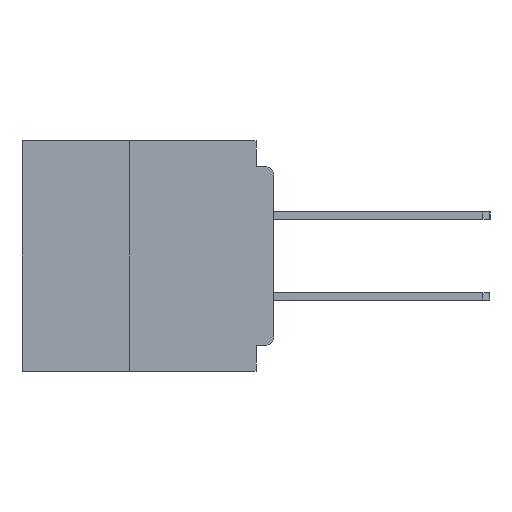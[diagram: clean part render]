
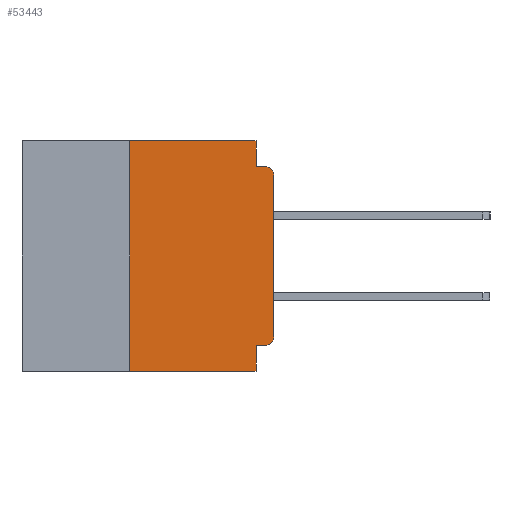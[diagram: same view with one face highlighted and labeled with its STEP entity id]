
A CAD part, left-side view. The second image highlights one B-rep face of the part: STEP entity #53443.
In plain terms, the highlighted planar face has unit normal (-1, 0, 0).
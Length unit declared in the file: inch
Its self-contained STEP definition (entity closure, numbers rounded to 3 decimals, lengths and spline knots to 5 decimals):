
#394 = VECTOR ( 'NONE', #37927, 39.37008 ) ;
#3602 = EDGE_CURVE ( 'NONE', #53124, #41101, #30416, .T. ) ;
#3615 = VECTOR ( 'NONE', #16809, 39.37008 ) ;
#4564 = PLANE ( 'NONE',  #59896 ) ;
#5155 = DIRECTION ( 'NONE',  ( 0., 0., 1. ) ) ;
#5938 = AXIS2_PLACEMENT_3D ( 'NONE', #44408, #13961, #49555 ) ;
#7149 = ORIENTED_EDGE ( 'NONE', *, *, #55955, .F. ) ;
#7468 = ORIENTED_EDGE ( 'NONE', *, *, #63781, .F. ) ;
#8582 = LINE ( 'NONE', #30007, #11817 ) ;
#8598 = VECTOR ( 'NONE', #38823, 39.37008 ) ;
#8826 = EDGE_CURVE ( 'NONE', #54804, #32072, #51766, .T. ) ;
#9048 = EDGE_CURVE ( 'NONE', #41101, #62053, #10284, .T. ) ;
#9780 = CARTESIAN_POINT ( 'NONE',  ( 0., 0.031, -0.355 ) ) ;
#10227 = LINE ( 'NONE', #23734, #8598 ) ;
#10284 = CIRCLE ( 'NONE', #5938, 0.015 ) ;
#11650 = CARTESIAN_POINT ( 'NONE',  ( 0., 0., -0.045 ) ) ;
#11817 = VECTOR ( 'NONE', #65470, 39.37008 ) ;
#11975 = ORIENTED_EDGE ( 'NONE', *, *, #19050, .F. ) ;
#13444 = CARTESIAN_POINT ( 'NONE',  ( 0., 0.031, -0.4 ) ) ;
#13961 = DIRECTION ( 'NONE',  ( -1., 0., 0. ) ) ;
#16021 = ORIENTED_EDGE ( 'NONE', *, *, #52593, .F. ) ;
#16647 = CARTESIAN_POINT ( 'NONE',  ( 0., 0.25, 0. ) ) ;
#16809 = DIRECTION ( 'NONE',  ( 0., -1., 0. ) ) ;
#16844 = VECTOR ( 'NONE', #5155, 39.37008 ) ;
#17705 = CARTESIAN_POINT ( 'NONE',  ( 0., 0.015, -0.34 ) ) ;
#19050 = EDGE_CURVE ( 'NONE', #55269, #35301, #8582, .T. ) ;
#22623 = ORIENTED_EDGE ( 'NONE', *, *, #8826, .T. ) ;
#22853 = DIRECTION ( 'NONE',  ( 0., 0., -1. ) ) ;
#23224 = ORIENTED_EDGE ( 'NONE', *, *, #56263, .F. ) ;
#23734 = CARTESIAN_POINT ( 'NONE',  ( 0., 0.031, 0. ) ) ;
#25204 = DIRECTION ( 'NONE',  ( 1., 0., 0. ) ) ;
#26945 = DIRECTION ( 'NONE',  ( 0., -1., 0. ) ) ;
#28700 = ORIENTED_EDGE ( 'NONE', *, *, #57626, .T. ) ;
#28778 = CARTESIAN_POINT ( 'NONE',  ( 0., 0.031, 0. ) ) ;
#29276 = ORIENTED_EDGE ( 'NONE', *, *, #52467, .F. ) ;
#30007 = CARTESIAN_POINT ( 'NONE',  ( 0., 0., -0.355 ) ) ;
#30416 = LINE ( 'NONE', #55993, #16844 ) ;
#30846 = LINE ( 'NONE', #11650, #3615 ) ;
#31445 = CARTESIAN_POINT ( 'NONE',  ( 0., 0.015, -0.045 ) ) ;
#31579 = CARTESIAN_POINT ( 'NONE',  ( 0., 0., -0.06 ) ) ;
#32072 = VERTEX_POINT ( 'NONE', #13444 ) ;
#32829 = CARTESIAN_POINT ( 'NONE',  ( 0., 0.25, -0.4 ) ) ;
#34481 = VERTEX_POINT ( 'NONE', #64232 ) ;
#35301 = VERTEX_POINT ( 'NONE', #9780 ) ;
#37617 = LINE ( 'NONE', #61578, #49532 ) ;
#37927 = DIRECTION ( 'NONE',  ( 0., 0., 1. ) ) ;
#37977 = LINE ( 'NONE', #32829, #394 ) ;
#38823 = DIRECTION ( 'NONE',  ( 0., 0., -1. ) ) ;
#41101 = VERTEX_POINT ( 'NONE', #31579 ) ;
#41611 = VECTOR ( 'NONE', #58799, 39.37008 ) ;
#42228 = CARTESIAN_POINT ( 'NONE',  ( 0., 0.437, -0.4 ) ) ;
#44310 = AXIS2_PLACEMENT_3D ( 'NONE', #17705, #53309, #22853 ) ;
#44408 = CARTESIAN_POINT ( 'NONE',  ( 0., 0.015, -0.06 ) ) ;
#44816 = VERTEX_POINT ( 'NONE', #16647 ) ;
#46308 = DIRECTION ( 'NONE',  ( 0., -1., 0. ) ) ;
#48862 = VERTEX_POINT ( 'NONE', #28778 ) ;
#49532 = VECTOR ( 'NONE', #46308, 39.37008 ) ;
#49555 = DIRECTION ( 'NONE',  ( 0., 0., -1. ) ) ;
#51372 = FACE_OUTER_BOUND ( 'NONE', #62338, .T. ) ;
#51766 = LINE ( 'NONE', #42228, #65213 ) ;
#52467 = EDGE_CURVE ( 'NONE', #34481, #62053, #30846, .T. ) ;
#52593 = EDGE_CURVE ( 'NONE', #54804, #44816, #37977, .T. ) ;
#53124 = VERTEX_POINT ( 'NONE', #53235 ) ;
#53235 = CARTESIAN_POINT ( 'NONE',  ( 0., 0., -0.34 ) ) ;
#53309 = DIRECTION ( 'NONE',  ( -1., 0., 0. ) ) ;
#53377 = CARTESIAN_POINT ( 'NONE',  ( 0., 0.015, -0.355 ) ) ;
#53443 = ADVANCED_FACE ( 'NONE', ( #51372 ), #4564, .F. ) ;
#53732 = CARTESIAN_POINT ( 'NONE',  ( 0., 0.031, -0.4 ) ) ;
#54699 = ORIENTED_EDGE ( 'NONE', *, *, #9048, .T. ) ;
#54804 = VERTEX_POINT ( 'NONE', #56774 ) ;
#55163 = LINE ( 'NONE', #53732, #41611 ) ;
#55269 = VERTEX_POINT ( 'NONE', #53377 ) ;
#55626 = CARTESIAN_POINT ( 'NONE',  ( 0., 0.437, 0. ) ) ;
#55955 = EDGE_CURVE ( 'NONE', #35301, #32072, #55163, .T. ) ;
#55993 = CARTESIAN_POINT ( 'NONE',  ( 0., 0., 0. ) ) ;
#56263 = EDGE_CURVE ( 'NONE', #44816, #48862, #37617, .T. ) ;
#56774 = CARTESIAN_POINT ( 'NONE',  ( 0., 0.25, -0.4 ) ) ;
#57626 = EDGE_CURVE ( 'NONE', #55269, #53124, #62788, .T. ) ;
#58799 = DIRECTION ( 'NONE',  ( 0., 0., -1. ) ) ;
#59896 = AXIS2_PLACEMENT_3D ( 'NONE', #55626, #25204, #60673 ) ;
#60195 = ORIENTED_EDGE ( 'NONE', *, *, #3602, .T. ) ;
#60673 = DIRECTION ( 'NONE',  ( 0., 0., -1. ) ) ;
#61578 = CARTESIAN_POINT ( 'NONE',  ( 0., 0.437, 0. ) ) ;
#62053 = VERTEX_POINT ( 'NONE', #31445 ) ;
#62338 = EDGE_LOOP ( 'NONE', ( #60195, #54699, #29276, #7468, #23224, #16021, #22623, #7149, #11975, #28700 ) ) ;
#62788 = CIRCLE ( 'NONE', #44310, 0.015 ) ;
#63781 = EDGE_CURVE ( 'NONE', #48862, #34481, #10227, .T. ) ;
#64232 = CARTESIAN_POINT ( 'NONE',  ( 0., 0.031, -0.045 ) ) ;
#65213 = VECTOR ( 'NONE', #26945, 39.37008 ) ;
#65470 = DIRECTION ( 'NONE',  ( 0., 1., 0. ) ) ;
